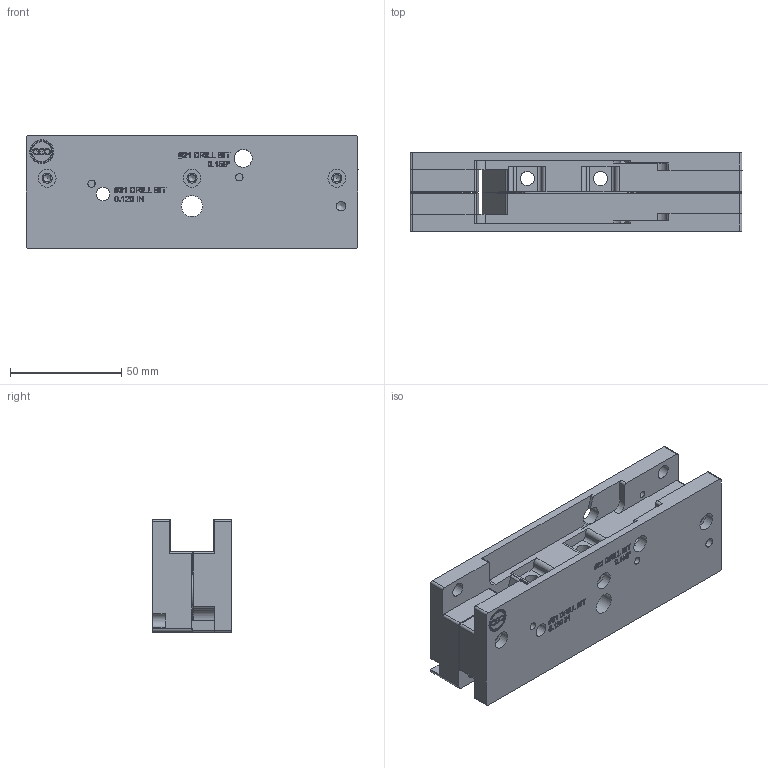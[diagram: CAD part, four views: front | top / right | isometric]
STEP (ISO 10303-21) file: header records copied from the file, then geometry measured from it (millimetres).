
FILE_DESCRIPTION(/* description */ (''),/* implementation_level */ '2;1');
FILE_NAME(/* name */ 'G80 FIXTURE REV E.step',/* time_stamp */ '2025-05-27T12:19:52-05:00',/* author */ (''),/* organization */ (''),/* preprocessor_version */ 'ST-DEVELOPER v20.1',/* originating_system */ 'Autodesk Translation Framework v14.10.0.0',/* authorisation */ '');
FILE_SCHEMA (('AUTOMOTIVE_DESIGN { 1 0 10303 214 3 1 1 }'));
Products named in the file (2): G80 FIXTURE REV E (Anodized); Component7
Assembly tree (1 placements, depth 2):
  G80 FIXTURE REV E (Anodized)
    Component7
Bounding box: 149.22 x 35.4 x 50.8 mm (x, y, z)
Volume: 189400.1 mm3; surface area: 51374.5 mm2
Topology: 2 solids, 2 shells, 1433 faces, 3932 edges, 2619 vertices
Faces by surface type: plane 704, bspline 637, cylinder 87, cone 5
Full cylindrical faces by diameter (mm): 2.997 x4, 3.332 x7, 4.234 x2, 4.5 x3, 6.071 x2, 6.401 x6, 8 x3, 8.077 x2, 9.525 x2
Entity records: 50801 total; most frequent: CARTESIAN_POINT 18623, ORIENTED_EDGE 7854, DIRECTION 4445, EDGE_CURVE 3927, VERTEX_POINT 2619, LINE 2459, VECTOR 2459, EDGE_LOOP 1584
